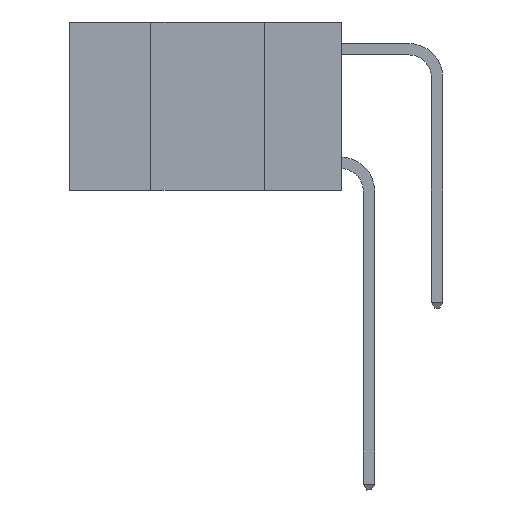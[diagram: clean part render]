
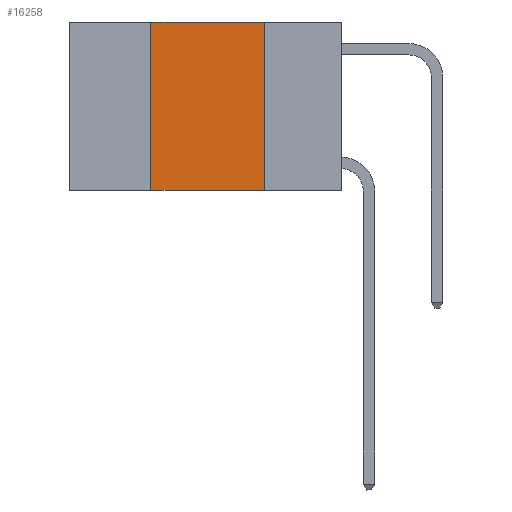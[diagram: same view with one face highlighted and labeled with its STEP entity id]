
A CAD part, left-side view. The second image highlights one B-rep face of the part: STEP entity #16258.
In plain terms, the highlighted planar face has unit normal (-1, 0, 0).
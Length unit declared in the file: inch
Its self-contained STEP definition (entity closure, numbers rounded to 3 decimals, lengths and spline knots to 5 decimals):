
#284 = EDGE_CURVE ( 'NONE', #2639, #10766, #12666, .T. ) ;
#567 = DIRECTION ( 'NONE',  ( 0., -1., 0. ) ) ;
#701 = ORIENTED_EDGE ( 'NONE', *, *, #284, .T. ) ;
#2639 = VERTEX_POINT ( 'NONE', #10090 ) ;
#3139 = ORIENTED_EDGE ( 'NONE', *, *, #13115, .F. ) ;
#3401 = VECTOR ( 'NONE', #567, 39.37008 ) ;
#4362 = CARTESIAN_POINT ( 'NONE',  ( 0., 0.6, 0. ) ) ;
#6405 = VECTOR ( 'NONE', #16141, 39.37008 ) ;
#6622 = CARTESIAN_POINT ( 'NONE',  ( 0., 0.17, -0.37 ) ) ;
#6944 = AXIS2_PLACEMENT_3D ( 'NONE', #19011, #20871, #10756 ) ;
#7962 = CARTESIAN_POINT ( 'NONE',  ( 0., 0.6, -0.37 ) ) ;
#8098 = VECTOR ( 'NONE', #19131, 39.37008 ) ;
#8616 = ORIENTED_EDGE ( 'NONE', *, *, #18436, .F. ) ;
#9163 = CARTESIAN_POINT ( 'NONE',  ( 0., 0.17, 0. ) ) ;
#9603 = LINE ( 'NONE', #14600, #12870 ) ;
#9709 = DIRECTION ( 'NONE',  ( 0., 0., -1. ) ) ;
#10090 = CARTESIAN_POINT ( 'NONE',  ( 0., 0.42, -0.37 ) ) ;
#10756 = DIRECTION ( 'NONE',  ( 0., 0., -1. ) ) ;
#10766 = VERTEX_POINT ( 'NONE', #6622 ) ;
#12567 = ORIENTED_EDGE ( 'NONE', *, *, #21311, .F. ) ;
#12642 = VERTEX_POINT ( 'NONE', #17531 ) ;
#12666 = LINE ( 'NONE', #7962, #6405 ) ;
#12870 = VECTOR ( 'NONE', #9709, 39.37008 ) ;
#13115 = EDGE_CURVE ( 'NONE', #12642, #13971, #14035, .T. ) ;
#13971 = VERTEX_POINT ( 'NONE', #9163 ) ;
#14035 = LINE ( 'NONE', #4362, #3401 ) ;
#14600 = CARTESIAN_POINT ( 'NONE',  ( 0., 0.17, 0. ) ) ;
#15659 = CARTESIAN_POINT ( 'NONE',  ( 0., 0.42, 0. ) ) ;
#16141 = DIRECTION ( 'NONE',  ( 0., -1., 0. ) ) ;
#16258 = ADVANCED_FACE ( 'NONE', ( #17591 ), #17160, .F. ) ;
#17160 = PLANE ( 'NONE',  #6944 ) ;
#17394 = LINE ( 'NONE', #15659, #8098 ) ;
#17531 = CARTESIAN_POINT ( 'NONE',  ( 0., 0.42, 0. ) ) ;
#17591 = FACE_OUTER_BOUND ( 'NONE', #17804, .T. ) ;
#17804 = EDGE_LOOP ( 'NONE', ( #8616, #3139, #12567, #701 ) ) ;
#18436 = EDGE_CURVE ( 'NONE', #13971, #10766, #9603, .T. ) ;
#19011 = CARTESIAN_POINT ( 'NONE',  ( 0., 0.6, 0. ) ) ;
#19131 = DIRECTION ( 'NONE',  ( 0., 0., 1. ) ) ;
#20871 = DIRECTION ( 'NONE',  ( 1., 0., 0. ) ) ;
#21311 = EDGE_CURVE ( 'NONE', #2639, #12642, #17394, .T. ) ;
